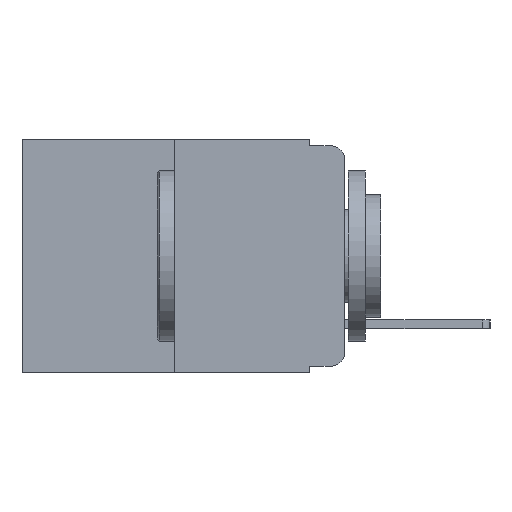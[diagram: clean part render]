
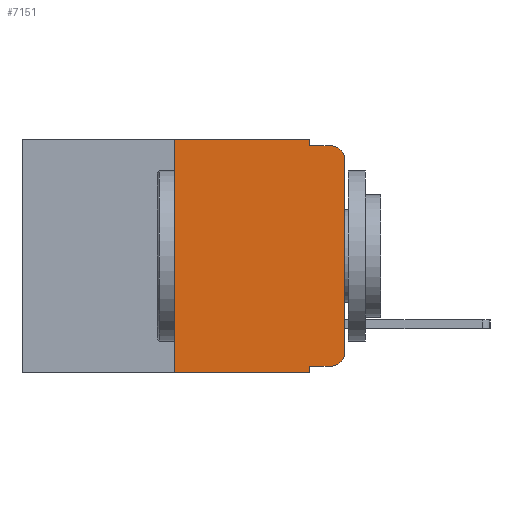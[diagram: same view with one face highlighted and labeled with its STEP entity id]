
A CAD part, left-side view. The second image highlights one B-rep face of the part: STEP entity #7151.
In plain terms, the highlighted planar face has unit normal (-1, 0, 0).
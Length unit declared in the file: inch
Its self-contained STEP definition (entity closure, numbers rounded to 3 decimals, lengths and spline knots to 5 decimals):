
#54 = ORIENTED_EDGE ( 'NONE', *, *, #11542, .T. ) ;
#67 = AXIS2_PLACEMENT_3D ( 'NONE', #12522, #12509, #11454 ) ;
#94 = VECTOR ( 'NONE', #5344, 39.37008 ) ;
#784 = VERTEX_POINT ( 'NONE', #9368 ) ;
#964 = CARTESIAN_POINT ( 'NONE',  ( 0., 0.25, 0. ) ) ;
#1169 = CIRCLE ( 'NONE', #4044, 0.02 ) ;
#1177 = DIRECTION ( 'NONE',  ( 0., -1., 0. ) ) ;
#1674 = AXIS2_PLACEMENT_3D ( 'NONE', #4928, #3864, #10850 ) ;
#1849 = EDGE_CURVE ( 'NONE', #3079, #8750, #8633, .T. ) ;
#2112 = CARTESIAN_POINT ( 'NONE',  ( 0., 0.473, -0.343 ) ) ;
#2373 = EDGE_CURVE ( 'NONE', #784, #6092, #8618, .T. ) ;
#2444 = ORIENTED_EDGE ( 'NONE', *, *, #10826, .F. ) ;
#2524 = EDGE_LOOP ( 'NONE', ( #9532, #12418, #2619, #2444, #4915, #13313, #3345, #9396, #12276, #54 ) ) ;
#2619 = ORIENTED_EDGE ( 'NONE', *, *, #2373, .F. ) ;
#2890 = CARTESIAN_POINT ( 'NONE',  ( 0., 0., -0.03 ) ) ;
#3003 = CARTESIAN_POINT ( 'NONE',  ( 0., 0.02, -0.01 ) ) ;
#3079 = VERTEX_POINT ( 'NONE', #5531 ) ;
#3133 = EDGE_CURVE ( 'NONE', #4991, #6092, #11212, .T. ) ;
#3235 = CARTESIAN_POINT ( 'NONE',  ( 0., 0.02, -0.313 ) ) ;
#3345 = ORIENTED_EDGE ( 'NONE', *, *, #7949, .T. ) ;
#3482 = CARTESIAN_POINT ( 'NONE',  ( 0., 0.25, -0.343 ) ) ;
#3864 = DIRECTION ( 'NONE',  ( 1., 0., 0. ) ) ;
#3879 = CARTESIAN_POINT ( 'NONE',  ( 0., 0.02, -0.333 ) ) ;
#4001 = LINE ( 'NONE', #2112, #9341 ) ;
#4044 = AXIS2_PLACEMENT_3D ( 'NONE', #3235, #10318, #4367 ) ;
#4178 = VERTEX_POINT ( 'NONE', #7085 ) ;
#4364 = DIRECTION ( 'NONE',  ( 0., -1., 0. ) ) ;
#4367 = DIRECTION ( 'NONE',  ( 0., 0., -1. ) ) ;
#4546 = LINE ( 'NONE', #964, #6872 ) ;
#4915 = ORIENTED_EDGE ( 'NONE', *, *, #13202, .F. ) ;
#4928 = CARTESIAN_POINT ( 'NONE',  ( 0., 0.473, 0. ) ) ;
#4991 = VERTEX_POINT ( 'NONE', #2890 ) ;
#5189 = VERTEX_POINT ( 'NONE', #10393 ) ;
#5213 = CARTESIAN_POINT ( 'NONE',  ( 0., 0.051, 0. ) ) ;
#5344 = DIRECTION ( 'NONE',  ( 0., 0., -1. ) ) ;
#5531 = CARTESIAN_POINT ( 'NONE',  ( 0., 0.051, -0.333 ) ) ;
#5808 = DIRECTION ( 'NONE',  ( 0., 0., 1. ) ) ;
#5967 = EDGE_CURVE ( 'NONE', #4178, #4991, #10123, .T. ) ;
#5992 = VERTEX_POINT ( 'NONE', #12711 ) ;
#6026 = CARTESIAN_POINT ( 'NONE',  ( 0., 0.473, 0. ) ) ;
#6092 = VERTEX_POINT ( 'NONE', #3003 ) ;
#6105 = FACE_OUTER_BOUND ( 'NONE', #2524, .T. ) ;
#6189 = DIRECTION ( 'NONE',  ( 0., 0., -1. ) ) ;
#6223 = VECTOR ( 'NONE', #12892, 39.37008 ) ;
#6349 = CARTESIAN_POINT ( 'NONE',  ( 0., 0.051, -0.01 ) ) ;
#6425 = DIRECTION ( 'NONE',  ( 0., -1., 0. ) ) ;
#6864 = EDGE_CURVE ( 'NONE', #9280, #5992, #4546, .T. ) ;
#6872 = VECTOR ( 'NONE', #7380, 39.37008 ) ;
#7085 = CARTESIAN_POINT ( 'NONE',  ( 0., 0., -0.313 ) ) ;
#7151 = ADVANCED_FACE ( 'NONE', ( #6105 ), #9898, .F. ) ;
#7345 = VECTOR ( 'NONE', #1177, 39.37008 ) ;
#7380 = DIRECTION ( 'NONE',  ( 0., 0., 1. ) ) ;
#7949 = EDGE_CURVE ( 'NONE', #9280, #8750, #4001, .T. ) ;
#7988 = VECTOR ( 'NONE', #6425, 39.37008 ) ;
#8305 = VECTOR ( 'NONE', #6189, 39.37008 ) ;
#8569 = CARTESIAN_POINT ( 'NONE',  ( 0., 0.051, -0.333 ) ) ;
#8618 = LINE ( 'NONE', #6349, #7988 ) ;
#8632 = LINE ( 'NONE', #5213, #8305 ) ;
#8633 = LINE ( 'NONE', #13410, #94 ) ;
#8750 = VERTEX_POINT ( 'NONE', #11510 ) ;
#8833 = LINE ( 'NONE', #6026, #6223 ) ;
#9280 = VERTEX_POINT ( 'NONE', #3482 ) ;
#9341 = VECTOR ( 'NONE', #4364, 39.37008 ) ;
#9368 = CARTESIAN_POINT ( 'NONE',  ( 0., 0.051, -0.01 ) ) ;
#9396 = ORIENTED_EDGE ( 'NONE', *, *, #1849, .F. ) ;
#9532 = ORIENTED_EDGE ( 'NONE', *, *, #5967, .T. ) ;
#9898 = PLANE ( 'NONE',  #1674 ) ;
#10123 = LINE ( 'NONE', #12668, #12988 ) ;
#10318 = DIRECTION ( 'NONE',  ( -1., 0., 0. ) ) ;
#10393 = CARTESIAN_POINT ( 'NONE',  ( 0., 0.051, 0. ) ) ;
#10826 = EDGE_CURVE ( 'NONE', #5189, #784, #8632, .T. ) ;
#10850 = DIRECTION ( 'NONE',  ( 0., 0., -1. ) ) ;
#11212 = CIRCLE ( 'NONE', #67, 0.02 ) ;
#11282 = VERTEX_POINT ( 'NONE', #3879 ) ;
#11454 = DIRECTION ( 'NONE',  ( 0., 0., -1. ) ) ;
#11510 = CARTESIAN_POINT ( 'NONE',  ( 0., 0.051, -0.343 ) ) ;
#11542 = EDGE_CURVE ( 'NONE', #11282, #4178, #1169, .T. ) ;
#11722 = EDGE_CURVE ( 'NONE', #3079, #11282, #12899, .T. ) ;
#12276 = ORIENTED_EDGE ( 'NONE', *, *, #11722, .T. ) ;
#12418 = ORIENTED_EDGE ( 'NONE', *, *, #3133, .T. ) ;
#12509 = DIRECTION ( 'NONE',  ( -1., 0., 0. ) ) ;
#12522 = CARTESIAN_POINT ( 'NONE',  ( 0., 0.02, -0.03 ) ) ;
#12668 = CARTESIAN_POINT ( 'NONE',  ( 0., 0., 0. ) ) ;
#12711 = CARTESIAN_POINT ( 'NONE',  ( 0., 0.25, 0. ) ) ;
#12892 = DIRECTION ( 'NONE',  ( 0., -1., 0. ) ) ;
#12899 = LINE ( 'NONE', #8569, #7345 ) ;
#12988 = VECTOR ( 'NONE', #5808, 39.37008 ) ;
#13202 = EDGE_CURVE ( 'NONE', #5992, #5189, #8833, .T. ) ;
#13313 = ORIENTED_EDGE ( 'NONE', *, *, #6864, .F. ) ;
#13410 = CARTESIAN_POINT ( 'NONE',  ( 0., 0.051, 0. ) ) ;
